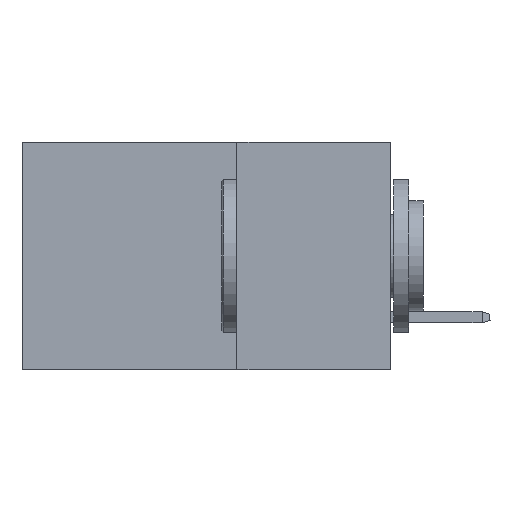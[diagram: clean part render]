
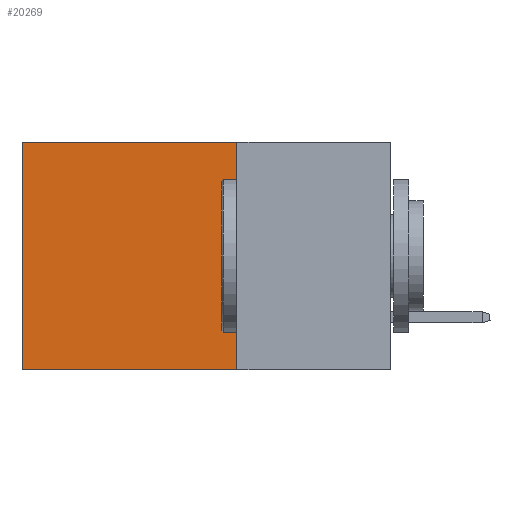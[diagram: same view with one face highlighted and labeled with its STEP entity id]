
A CAD part, left-side view. The second image highlights one B-rep face of the part: STEP entity #20269.
In plain terms, the highlighted planar face has unit normal (-1, 0, 0).
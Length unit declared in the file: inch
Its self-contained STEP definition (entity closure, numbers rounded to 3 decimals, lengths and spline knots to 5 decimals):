
#82 = CARTESIAN_POINT ( 'NONE',  ( 0.2875, 0.25, -0.37 ) ) ;
#5342 = LINE ( 'NONE', #15976, #17990 ) ;
#6509 = FACE_OUTER_BOUND ( 'NONE', #35155, .T. ) ;
#6866 = DIRECTION ( 'NONE',  ( 0., 0., -1. ) ) ;
#7224 = CARTESIAN_POINT ( 'NONE',  ( 0.2875, 0.6, 0. ) ) ;
#9244 = LINE ( 'NONE', #39803, #31169 ) ;
#12234 = VECTOR ( 'NONE', #31315, 39.37008 ) ;
#13368 = VECTOR ( 'NONE', #14900, 39.37008 ) ;
#14900 = DIRECTION ( 'NONE',  ( 0., 1., 0. ) ) ;
#15373 = ORIENTED_EDGE ( 'NONE', *, *, #33668, .T. ) ;
#15399 = EDGE_CURVE ( 'NONE', #36269, #20554, #36338, .T. ) ;
#15976 = CARTESIAN_POINT ( 'NONE',  ( 0.2875, 0.6, 0. ) ) ;
#16113 = CARTESIAN_POINT ( 'NONE',  ( 0.2875, 0.25, 0. ) ) ;
#17990 = VECTOR ( 'NONE', #21587, 39.37008 ) ;
#19259 = DIRECTION ( 'NONE',  ( 1., 0., 0. ) ) ;
#20171 = ORIENTED_EDGE ( 'NONE', *, *, #39262, .F. ) ;
#20269 = ADVANCED_FACE ( 'NONE', ( #6509 ), #35068, .F. ) ;
#20554 = VERTEX_POINT ( 'NONE', #7224 ) ;
#21587 = DIRECTION ( 'NONE',  ( 0., 0., -1. ) ) ;
#22427 = LINE ( 'NONE', #82, #12234 ) ;
#22513 = VERTEX_POINT ( 'NONE', #23468 ) ;
#22838 = CARTESIAN_POINT ( 'NONE',  ( 0.2875, 0.25, 0. ) ) ;
#23468 = CARTESIAN_POINT ( 'NONE',  ( 0.2875, 0.6, -0.37 ) ) ;
#24203 = CARTESIAN_POINT ( 'NONE',  ( 0.2875, 0.25, 0. ) ) ;
#26485 = AXIS2_PLACEMENT_3D ( 'NONE', #16113, #19259, #6866 ) ;
#29148 = ORIENTED_EDGE ( 'NONE', *, *, #15399, .T. ) ;
#31169 = VECTOR ( 'NONE', #33725, 39.37008 ) ;
#31315 = DIRECTION ( 'NONE',  ( 0., 1., 0. ) ) ;
#31573 = VERTEX_POINT ( 'NONE', #34394 ) ;
#33668 = EDGE_CURVE ( 'NONE', #20554, #22513, #5342, .T. ) ;
#33725 = DIRECTION ( 'NONE',  ( 0., 0., -1. ) ) ;
#34394 = CARTESIAN_POINT ( 'NONE',  ( 0.2875, 0.25, -0.37 ) ) ;
#35068 = PLANE ( 'NONE',  #26485 ) ;
#35155 = EDGE_LOOP ( 'NONE', ( #15373, #36544, #20171, #29148 ) ) ;
#36269 = VERTEX_POINT ( 'NONE', #22838 ) ;
#36338 = LINE ( 'NONE', #24203, #13368 ) ;
#36544 = ORIENTED_EDGE ( 'NONE', *, *, #38646, .F. ) ;
#38646 = EDGE_CURVE ( 'NONE', #31573, #22513, #22427, .T. ) ;
#39262 = EDGE_CURVE ( 'NONE', #36269, #31573, #9244, .T. ) ;
#39803 = CARTESIAN_POINT ( 'NONE',  ( 0.2875, 0.25, 0. ) ) ;
